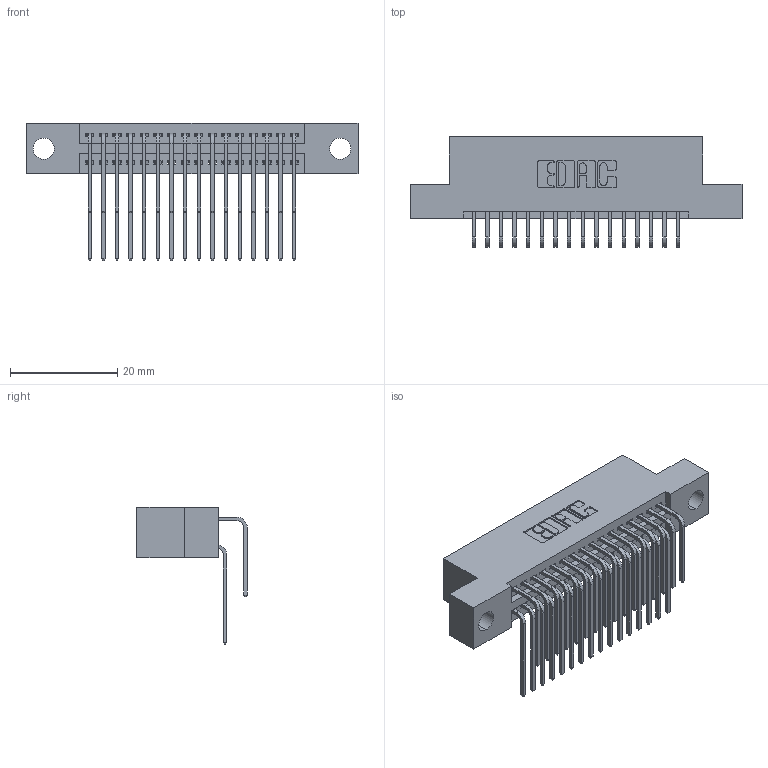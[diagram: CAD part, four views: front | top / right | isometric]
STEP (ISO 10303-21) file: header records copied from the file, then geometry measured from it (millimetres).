
FILE_DESCRIPTION (( 'STEP AP203' ), '1' );
FILE_NAME ('345-032-559-204.STEP', '2021-05-19T23:52:33', ( '' ), ( '' ), 'SwSTEP 2.0', 'SolidWorks 2020', '' );
FILE_SCHEMA (( 'CONFIG_CONTROL_DESIGN' ));
Length unit declared in the file: inch
Products named in the file (4): 345 Part_Flush Mounting Lugs - 0.156 Dia-TI; 345-292-001_559 Tail - 2; 345-292-001_558 559 Tail - 1; 345-032-559-204
Assembly tree (33 placements, depth 2):
  345-032-559-204
    345 Part_Flush Mounting Lugs - 0.156 Dia-TI
    345-292-001_558 559 Tail - 1  x16
    345-292-001_559 Tail - 2  x16
Bounding box: 61.85 x 20.56 x 25.53 mm (x, y, z)
Volume: 5845.4 mm3; surface area: 8856.5 mm2
Topology: 33 solids, 33 shells, 1804 faces, 5337 edges, 3514 vertices
Faces by surface type: plane 1214, cylinder 590
Entity records: 18125 total; most frequent: CARTESIAN_POINT 3113, ORIENTED_EDGE 2994, DIRECTION 2749, EDGE_CURVE 1497, LINE 1261, VECTOR 1261, VERTEX_POINT 994, AXIS2_PLACEMENT_3D 744
